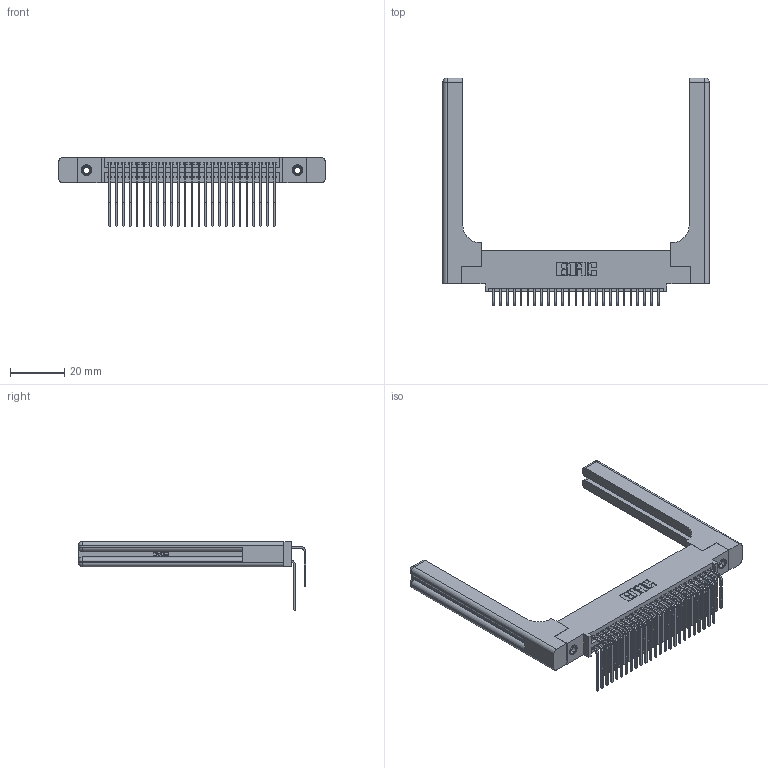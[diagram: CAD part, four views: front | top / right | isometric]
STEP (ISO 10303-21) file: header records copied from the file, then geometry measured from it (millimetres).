
FILE_DESCRIPTION (( 'STEP AP203' ), '1' );
FILE_NAME ('345-050-559-558.STEP', '2019-10-29T13:22:28', ( '' ), ( '' ), 'SwSTEP 2.0', 'SolidWorks 2016', '' );
FILE_SCHEMA (( 'CONFIG_CONTROL_DESIGN' ));
Length unit declared in the file: inch
Products named in the file (6): 345-250-001_345-250-001-102; 345-292-001_558 559 Tail - 1; 345-220-058_345-220-058; 345 Part_0.110 Offset - 0.156 Dia-TH; 345-050-559-558; 345-292-001_559 Tail - 2
Assembly tree (55 placements, depth 2):
  345-050-559-558
    345 Part_0.110 Offset - 0.156 Dia-TH
    345-292-001_558 559 Tail - 1  x25
    345-292-001_559 Tail - 2  x25
    345-250-001_345-250-001-102  x2
    345-220-058_345-220-058  x2
Bounding box: 98.53 x 84.32 x 25.53 mm (x, y, z)
Volume: 18103.4 mm3; surface area: 20410.9 mm2
Topology: 55 solids, 55 shells, 2986 faces, 8769 edges, 5758 vertices
Faces by surface type: plane 1982, cylinder 944, bspline 36, cone 12, sphere 8, torus 4
Entity records: 28870 total; most frequent: CARTESIAN_POINT 5896, ORIENTED_EDGE 4576, DIRECTION 4124, EDGE_CURVE 2288, VECTOR 1924, LINE 1924, VERTEX_POINT 1514, AXIS2_PLACEMENT_3D 1100
